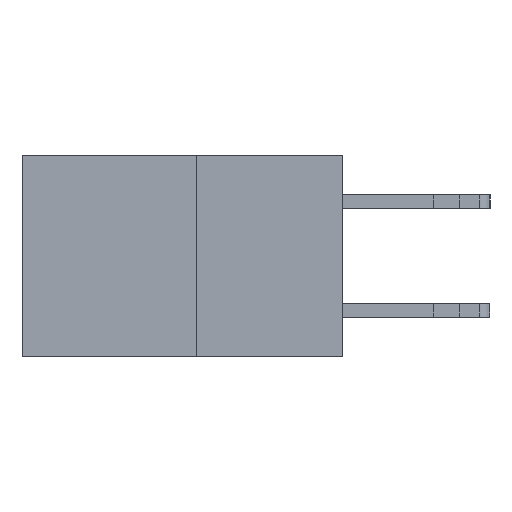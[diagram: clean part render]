
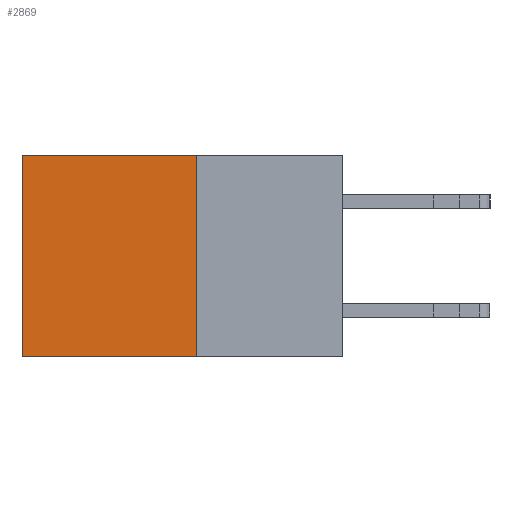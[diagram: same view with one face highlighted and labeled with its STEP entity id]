
A CAD part, left-side view. The second image highlights one B-rep face of the part: STEP entity #2869.
In plain terms, the highlighted planar face has unit normal (-1, 0, 0).
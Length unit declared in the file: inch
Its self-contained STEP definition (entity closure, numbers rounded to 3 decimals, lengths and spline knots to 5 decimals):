
#447 = EDGE_CURVE ( 'NONE', #6592, #14907, #1016, .T. ) ;
#531 = VECTOR ( 'NONE', #10644, 39.37008 ) ;
#680 = VECTOR ( 'NONE', #14415, 39.37008 ) ;
#1016 = LINE ( 'NONE', #5254, #531 ) ;
#1304 = CARTESIAN_POINT ( 'NONE',  ( 0.277, 0.27, 0. ) ) ;
#2480 = VERTEX_POINT ( 'NONE', #1304 ) ;
#2613 = EDGE_CURVE ( 'NONE', #2480, #6592, #16681, .T. ) ;
#2869 = ADVANCED_FACE ( 'NONE', ( #12546 ), #12222, .F. ) ;
#3044 = LINE ( 'NONE', #17764, #11125 ) ;
#3887 = EDGE_CURVE ( 'NONE', #2480, #7817, #3044, .T. ) ;
#4183 = CARTESIAN_POINT ( 'NONE',  ( 0.277, 0.59, 0. ) ) ;
#4594 = EDGE_CURVE ( 'NONE', #7817, #14907, #15780, .T. ) ;
#5254 = CARTESIAN_POINT ( 'NONE',  ( 0.277, 0.27, -0.37 ) ) ;
#5436 = DIRECTION ( 'NONE',  ( 0., 0., -1. ) ) ;
#6592 = VERTEX_POINT ( 'NONE', #14189 ) ;
#7511 = EDGE_LOOP ( 'NONE', ( #16037, #15575, #8662, #16961 ) ) ;
#7817 = VERTEX_POINT ( 'NONE', #4183 ) ;
#8662 = ORIENTED_EDGE ( 'NONE', *, *, #2613, .F. ) ;
#8863 = VECTOR ( 'NONE', #5436, 39.37008 ) ;
#10015 = DIRECTION ( 'NONE',  ( 0., 0., -1. ) ) ;
#10644 = DIRECTION ( 'NONE',  ( 0., 1., 0. ) ) ;
#10812 = DIRECTION ( 'NONE',  ( 1., 0., 0. ) ) ;
#10874 = CARTESIAN_POINT ( 'NONE',  ( 0.277, 0.27, -0.37 ) ) ;
#11125 = VECTOR ( 'NONE', #15984, 39.37008 ) ;
#11593 = CARTESIAN_POINT ( 'NONE',  ( 0.277, 0.27, -0.37 ) ) ;
#12222 = PLANE ( 'NONE',  #17195 ) ;
#12546 = FACE_OUTER_BOUND ( 'NONE', #7511, .T. ) ;
#14189 = CARTESIAN_POINT ( 'NONE',  ( 0.277, 0.27, -0.37 ) ) ;
#14386 = CARTESIAN_POINT ( 'NONE',  ( 0.277, 0.59, -0.37 ) ) ;
#14415 = DIRECTION ( 'NONE',  ( 0., 0., -1. ) ) ;
#14907 = VERTEX_POINT ( 'NONE', #19230 ) ;
#15575 = ORIENTED_EDGE ( 'NONE', *, *, #447, .F. ) ;
#15780 = LINE ( 'NONE', #14386, #8863 ) ;
#15984 = DIRECTION ( 'NONE',  ( 0., 1., 0. ) ) ;
#16037 = ORIENTED_EDGE ( 'NONE', *, *, #4594, .T. ) ;
#16681 = LINE ( 'NONE', #11593, #680 ) ;
#16961 = ORIENTED_EDGE ( 'NONE', *, *, #3887, .T. ) ;
#17195 = AXIS2_PLACEMENT_3D ( 'NONE', #10874, #10812, #10015 ) ;
#17764 = CARTESIAN_POINT ( 'NONE',  ( 0.277, 0.27, 0. ) ) ;
#19230 = CARTESIAN_POINT ( 'NONE',  ( 0.277, 0.59, -0.37 ) ) ;
